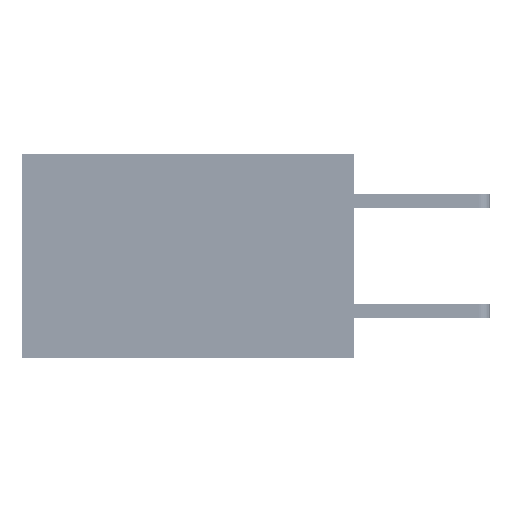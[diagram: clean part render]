
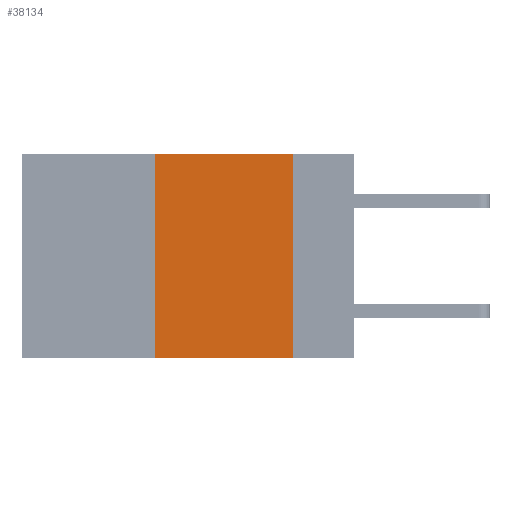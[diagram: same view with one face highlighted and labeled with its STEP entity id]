
A CAD part, left-side view. The second image highlights one B-rep face of the part: STEP entity #38134.
In plain terms, the highlighted planar face has unit normal (-1, 0, 0).
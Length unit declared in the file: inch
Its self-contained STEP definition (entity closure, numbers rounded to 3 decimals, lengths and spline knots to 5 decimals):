
#2769 = CARTESIAN_POINT ( 'NONE',  ( 0., 0.36, 0. ) ) ;
#2966 = DIRECTION ( 'NONE',  ( 0., -1., 0. ) ) ;
#4557 = DIRECTION ( 'NONE',  ( 1., 0., 0. ) ) ;
#7319 = CARTESIAN_POINT ( 'NONE',  ( 0., 0.6, 0. ) ) ;
#7377 = FACE_OUTER_BOUND ( 'NONE', #40559, .T. ) ;
#9453 = CARTESIAN_POINT ( 'NONE',  ( 0., 0.6, -0.37 ) ) ;
#9949 = LINE ( 'NONE', #9453, #32571 ) ;
#11297 = VERTEX_POINT ( 'NONE', #42476 ) ;
#15478 = VERTEX_POINT ( 'NONE', #2769 ) ;
#16023 = ORIENTED_EDGE ( 'NONE', *, *, #42189, .F. ) ;
#17872 = ORIENTED_EDGE ( 'NONE', *, *, #18729, .F. ) ;
#18729 = EDGE_CURVE ( 'NONE', #34072, #15478, #44046, .T. ) ;
#19075 = AXIS2_PLACEMENT_3D ( 'NONE', #23528, #4557, #30967 ) ;
#19135 = ORIENTED_EDGE ( 'NONE', *, *, #50005, .F. ) ;
#23528 = CARTESIAN_POINT ( 'NONE',  ( 0., 0.6, 0. ) ) ;
#25051 = VERTEX_POINT ( 'NONE', #36461 ) ;
#25919 = LINE ( 'NONE', #29258, #38769 ) ;
#29258 = CARTESIAN_POINT ( 'NONE',  ( 0., 0.11, 0. ) ) ;
#29301 = VECTOR ( 'NONE', #32014, 39.37008 ) ;
#30203 = VECTOR ( 'NONE', #2966, 39.37008 ) ;
#30967 = DIRECTION ( 'NONE',  ( 0., 0., -1. ) ) ;
#32014 = DIRECTION ( 'NONE',  ( 0., 0., 1. ) ) ;
#32571 = VECTOR ( 'NONE', #33533, 39.37008 ) ;
#33533 = DIRECTION ( 'NONE',  ( 0., -1., 0. ) ) ;
#34072 = VERTEX_POINT ( 'NONE', #47980 ) ;
#36461 = CARTESIAN_POINT ( 'NONE',  ( 0., 0.11, -0.37 ) ) ;
#38134 = ADVANCED_FACE ( 'NONE', ( #7377 ), #39921, .F. ) ;
#38769 = VECTOR ( 'NONE', #40791, 39.37008 ) ;
#38827 = LINE ( 'NONE', #7319, #30203 ) ;
#39921 = PLANE ( 'NONE',  #19075 ) ;
#40559 = EDGE_LOOP ( 'NONE', ( #16023, #19135, #17872, #48475 ) ) ;
#40791 = DIRECTION ( 'NONE',  ( 0., 0., -1. ) ) ;
#42189 = EDGE_CURVE ( 'NONE', #11297, #25051, #25919, .T. ) ;
#42476 = CARTESIAN_POINT ( 'NONE',  ( 0., 0.11, 0. ) ) ;
#44046 = LINE ( 'NONE', #47382, #29301 ) ;
#46588 = EDGE_CURVE ( 'NONE', #34072, #25051, #9949, .T. ) ;
#47382 = CARTESIAN_POINT ( 'NONE',  ( 0., 0.36, 0. ) ) ;
#47980 = CARTESIAN_POINT ( 'NONE',  ( 0., 0.36, -0.37 ) ) ;
#48475 = ORIENTED_EDGE ( 'NONE', *, *, #46588, .T. ) ;
#50005 = EDGE_CURVE ( 'NONE', #15478, #11297, #38827, .T. ) ;
